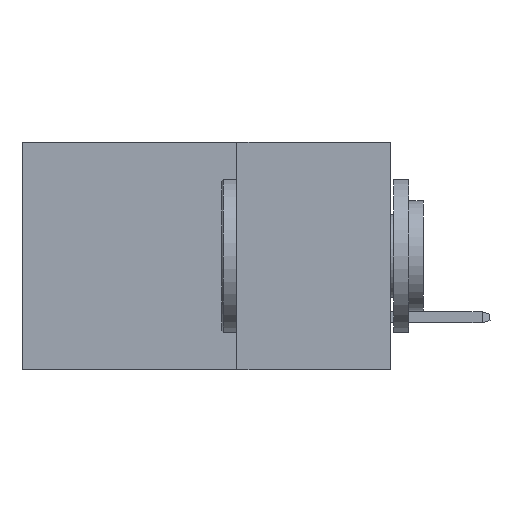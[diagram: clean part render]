
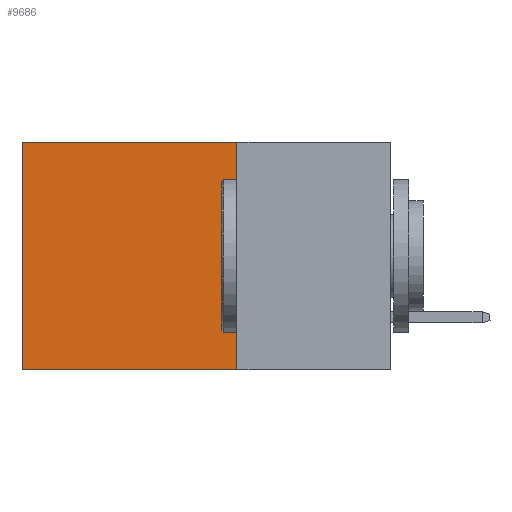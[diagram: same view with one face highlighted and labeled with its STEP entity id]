
A CAD part, left-side view. The second image highlights one B-rep face of the part: STEP entity #9686.
In plain terms, the highlighted planar face has unit normal (-1, 0, 0).
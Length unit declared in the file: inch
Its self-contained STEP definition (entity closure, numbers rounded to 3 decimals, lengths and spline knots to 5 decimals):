
#530 = ORIENTED_EDGE ( 'NONE', *, *, #9139, .T. ) ;
#536 = VECTOR ( 'NONE', #2778, 39.37008 ) ;
#596 = LINE ( 'NONE', #5744, #7612 ) ;
#790 = VECTOR ( 'NONE', #8091, 39.37008 ) ;
#907 = CARTESIAN_POINT ( 'NONE',  ( 0.2875, 0.6, 0. ) ) ;
#1321 = VERTEX_POINT ( 'NONE', #907 ) ;
#1429 = LINE ( 'NONE', #10706, #790 ) ;
#1486 = DIRECTION ( 'NONE',  ( 0., 0., -1. ) ) ;
#2266 = VERTEX_POINT ( 'NONE', #9406 ) ;
#2444 = ORIENTED_EDGE ( 'NONE', *, *, #4492, .F. ) ;
#2778 = DIRECTION ( 'NONE',  ( 0., 0., -1. ) ) ;
#3134 = LINE ( 'NONE', #7770, #7756 ) ;
#3813 = CARTESIAN_POINT ( 'NONE',  ( 0.2875, 0.6, 0. ) ) ;
#3919 = VERTEX_POINT ( 'NONE', #4115 ) ;
#4115 = CARTESIAN_POINT ( 'NONE',  ( 0.2875, 0.25, 0. ) ) ;
#4253 = FACE_OUTER_BOUND ( 'NONE', #5183, .T. ) ;
#4286 = EDGE_CURVE ( 'NONE', #7804, #2266, #596, .T. ) ;
#4321 = AXIS2_PLACEMENT_3D ( 'NONE', #4462, #7174, #1486 ) ;
#4462 = CARTESIAN_POINT ( 'NONE',  ( 0.2875, 0.25, 0. ) ) ;
#4492 = EDGE_CURVE ( 'NONE', #3919, #7804, #3134, .T. ) ;
#5183 = EDGE_LOOP ( 'NONE', ( #11599, #11199, #2444, #530 ) ) ;
#5744 = CARTESIAN_POINT ( 'NONE',  ( 0.2875, 0.25, -0.37 ) ) ;
#5876 = DIRECTION ( 'NONE',  ( 0., 1., 0. ) ) ;
#6003 = EDGE_CURVE ( 'NONE', #1321, #2266, #7563, .T. ) ;
#7174 = DIRECTION ( 'NONE',  ( 1., 0., 0. ) ) ;
#7563 = LINE ( 'NONE', #3813, #536 ) ;
#7612 = VECTOR ( 'NONE', #5876, 39.37008 ) ;
#7692 = DIRECTION ( 'NONE',  ( 0., 0., -1. ) ) ;
#7756 = VECTOR ( 'NONE', #7692, 39.37008 ) ;
#7770 = CARTESIAN_POINT ( 'NONE',  ( 0.2875, 0.25, 0. ) ) ;
#7804 = VERTEX_POINT ( 'NONE', #8987 ) ;
#8091 = DIRECTION ( 'NONE',  ( 0., 1., 0. ) ) ;
#8987 = CARTESIAN_POINT ( 'NONE',  ( 0.2875, 0.25, -0.37 ) ) ;
#9139 = EDGE_CURVE ( 'NONE', #3919, #1321, #1429, .T. ) ;
#9406 = CARTESIAN_POINT ( 'NONE',  ( 0.2875, 0.6, -0.37 ) ) ;
#9686 = ADVANCED_FACE ( 'NONE', ( #4253 ), #10650, .F. ) ;
#10650 = PLANE ( 'NONE',  #4321 ) ;
#10706 = CARTESIAN_POINT ( 'NONE',  ( 0.2875, 0.25, 0. ) ) ;
#11199 = ORIENTED_EDGE ( 'NONE', *, *, #4286, .F. ) ;
#11599 = ORIENTED_EDGE ( 'NONE', *, *, #6003, .T. ) ;
